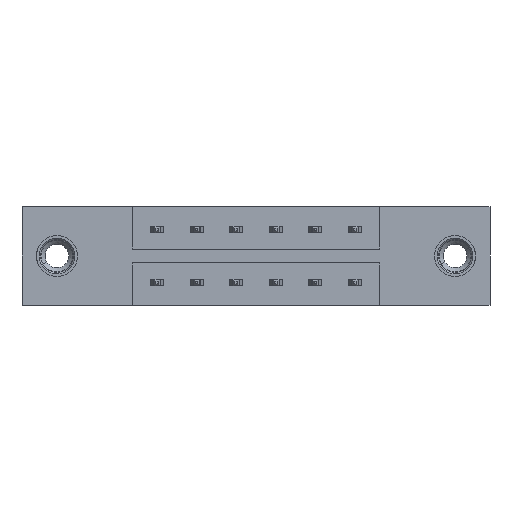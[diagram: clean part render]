
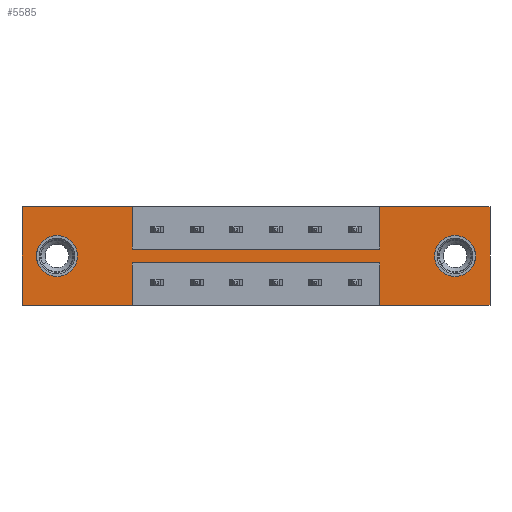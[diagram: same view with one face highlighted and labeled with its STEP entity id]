
A CAD part, front view. The second image highlights one B-rep face of the part: STEP entity #5585.
In plain terms, the highlighted planar face has unit normal (0, -1, 0).
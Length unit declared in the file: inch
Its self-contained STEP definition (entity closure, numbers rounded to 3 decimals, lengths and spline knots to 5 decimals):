
#4 = CARTESIAN_POINT ( 'NONE',  ( 1.775, 0., -0.375 ) ) ;
#118 = VERTEX_POINT ( 'NONE', #8989 ) ;
#135 = VECTOR ( 'NONE', #5515, 39.37008 ) ;
#169 = CIRCLE ( 'NONE', #7778, 0.078 ) ;
#213 = CARTESIAN_POINT ( 'NONE',  ( 0., 0., -0.375 ) ) ;
#219 = DIRECTION ( 'NONE',  ( 1., 0., 0. ) ) ;
#238 = VECTOR ( 'NONE', #4955, 39.37008 ) ;
#366 = DIRECTION ( 'NONE',  ( 0., 0., -1. ) ) ;
#485 = VECTOR ( 'NONE', #2483, 39.37008 ) ;
#530 = EDGE_CURVE ( 'NONE', #4576, #9027, #7301, .T. ) ;
#542 = ORIENTED_EDGE ( 'NONE', *, *, #5219, .F. ) ;
#544 = CARTESIAN_POINT ( 'NONE',  ( 1.6425, 0., -0.1875 ) ) ;
#625 = CARTESIAN_POINT ( 'NONE',  ( 0., 0., -0.375 ) ) ;
#694 = EDGE_CURVE ( 'NONE', #2834, #7868, #1300, .T. ) ;
#775 = CIRCLE ( 'NONE', #926, 0.078 ) ;
#806 = VERTEX_POINT ( 'NONE', #3602 ) ;
#830 = VECTOR ( 'NONE', #8016, 39.37008 ) ;
#875 = VECTOR ( 'NONE', #9648, 39.37008 ) ;
#926 = AXIS2_PLACEMENT_3D ( 'NONE', #544, #2720, #4322 ) ;
#1106 = AXIS2_PLACEMENT_3D ( 'NONE', #6571, #8780, #6470 ) ;
#1131 = ORIENTED_EDGE ( 'NONE', *, *, #530, .F. ) ;
#1161 = EDGE_LOOP ( 'NONE', ( #6562, #8916, #1131, #5868, #542, #4214, #4655, #4338, #6987, #3569, #9033, #2171 ) ) ;
#1178 = LINE ( 'NONE', #2723, #830 ) ;
#1208 = EDGE_CURVE ( 'NONE', #806, #8581, #5520, .T. ) ;
#1234 = EDGE_CURVE ( 'NONE', #5069, #4576, #1178, .T. ) ;
#1300 = LINE ( 'NONE', #625, #1649 ) ;
#1394 = VECTOR ( 'NONE', #366, 39.37008 ) ;
#1538 = VERTEX_POINT ( 'NONE', #7595 ) ;
#1649 = VECTOR ( 'NONE', #7380, 39.37008 ) ;
#1722 = CARTESIAN_POINT ( 'NONE',  ( 0., 0., 0. ) ) ;
#1952 = DIRECTION ( 'NONE',  ( 0., 1., 0. ) ) ;
#2171 = ORIENTED_EDGE ( 'NONE', *, *, #3201, .F. ) ;
#2472 = LINE ( 'NONE', #6971, #485 ) ;
#2483 = DIRECTION ( 'NONE',  ( 0., 0., 1. ) ) ;
#2505 = VERTEX_POINT ( 'NONE', #2828 ) ;
#2542 = VERTEX_POINT ( 'NONE', #7254 ) ;
#2720 = DIRECTION ( 'NONE',  ( 0., 1., 0. ) ) ;
#2723 = CARTESIAN_POINT ( 'NONE',  ( 0., 0., 0. ) ) ;
#2746 = LINE ( 'NONE', #4334, #5218 ) ;
#2828 = CARTESIAN_POINT ( 'NONE',  ( 1.6425, 0., -0.2655 ) ) ;
#2834 = VERTEX_POINT ( 'NONE', #4659 ) ;
#2861 = CARTESIAN_POINT ( 'NONE',  ( 1.775, 0., 0. ) ) ;
#2870 = LINE ( 'NONE', #9576, #875 ) ;
#2894 = AXIS2_PLACEMENT_3D ( 'NONE', #7270, #1952, #3412 ) ;
#2920 = AXIS2_PLACEMENT_3D ( 'NONE', #213, #7633, #7694 ) ;
#2939 = EDGE_CURVE ( 'NONE', #6679, #9699, #7095, .T. ) ;
#3072 = CARTESIAN_POINT ( 'NONE',  ( 0.4175, 0., 0. ) ) ;
#3193 = EDGE_CURVE ( 'NONE', #118, #2542, #2870, .T. ) ;
#3201 = EDGE_CURVE ( 'NONE', #2542, #4080, #5339, .T. ) ;
#3412 = DIRECTION ( 'NONE',  ( 0., 0., 1. ) ) ;
#3569 = ORIENTED_EDGE ( 'NONE', *, *, #694, .F. ) ;
#3581 = CARTESIAN_POINT ( 'NONE',  ( 0.4175, 0., -0.214 ) ) ;
#3602 = CARTESIAN_POINT ( 'NONE',  ( 0.1325, 0., -0.1095 ) ) ;
#3751 = EDGE_LOOP ( 'NONE', ( #9052, #9121 ) ) ;
#3846 = DIRECTION ( 'NONE',  ( 1., 0., 0. ) ) ;
#3864 = EDGE_CURVE ( 'NONE', #9699, #6518, #6841, .T. ) ;
#3989 = VERTEX_POINT ( 'NONE', #5786 ) ;
#4080 = VERTEX_POINT ( 'NONE', #4458 ) ;
#4113 = CARTESIAN_POINT ( 'NONE',  ( 1.775, 0., 0. ) ) ;
#4168 = DIRECTION ( 'NONE',  ( 0., 1., 0. ) ) ;
#4214 = ORIENTED_EDGE ( 'NONE', *, *, #7683, .F. ) ;
#4322 = DIRECTION ( 'NONE',  ( 0., 0., -1. ) ) ;
#4324 = VECTOR ( 'NONE', #3846, 39.37008 ) ;
#4334 = CARTESIAN_POINT ( 'NONE',  ( 0., 0., -0.375 ) ) ;
#4338 = ORIENTED_EDGE ( 'NONE', *, *, #2939, .F. ) ;
#4458 = CARTESIAN_POINT ( 'NONE',  ( 0.4175, 0., -0.214 ) ) ;
#4576 = VERTEX_POINT ( 'NONE', #2861 ) ;
#4655 = ORIENTED_EDGE ( 'NONE', *, *, #3864, .F. ) ;
#4659 = CARTESIAN_POINT ( 'NONE',  ( 0.4175, 0., -0.375 ) ) ;
#4712 = CARTESIAN_POINT ( 'NONE',  ( 0.1325, 0., -0.2655 ) ) ;
#4729 = CARTESIAN_POINT ( 'NONE',  ( 1.3575, 0., 0. ) ) ;
#4783 = EDGE_LOOP ( 'NONE', ( #7637, #8274 ) ) ;
#4851 = VECTOR ( 'NONE', #5842, 39.37008 ) ;
#4955 = DIRECTION ( 'NONE',  ( 0., 0., 1. ) ) ;
#5042 = LINE ( 'NONE', #9327, #1394 ) ;
#5069 = VERTEX_POINT ( 'NONE', #4729 ) ;
#5081 = EDGE_CURVE ( 'NONE', #7868, #6679, #2472, .T. ) ;
#5143 = CARTESIAN_POINT ( 'NONE',  ( 0.4175, 0., -0.161 ) ) ;
#5189 = LINE ( 'NONE', #7246, #238 ) ;
#5218 = VECTOR ( 'NONE', #8197, 39.37008 ) ;
#5219 = EDGE_CURVE ( 'NONE', #1538, #5069, #5189, .T. ) ;
#5339 = LINE ( 'NONE', #3581, #7563 ) ;
#5515 = DIRECTION ( 'NONE',  ( 0., 0., -1. ) ) ;
#5520 = CIRCLE ( 'NONE', #2894, 0.078 ) ;
#5585 = ADVANCED_FACE ( 'NONE', ( #9280, #7155, #7861 ), #6870, .T. ) ;
#5786 = CARTESIAN_POINT ( 'NONE',  ( 1.6425, 0., -0.1095 ) ) ;
#5842 = DIRECTION ( 'NONE',  ( 0., 0., -1. ) ) ;
#5868 = ORIENTED_EDGE ( 'NONE', *, *, #1234, .F. ) ;
#6352 = EDGE_CURVE ( 'NONE', #4080, #2834, #5042, .T. ) ;
#6370 = CARTESIAN_POINT ( 'NONE',  ( 0.1325, 0., -0.1875 ) ) ;
#6443 = DIRECTION ( 'NONE',  ( 0., 0., 1. ) ) ;
#6470 = DIRECTION ( 'NONE',  ( 0., 0., -1. ) ) ;
#6506 = DIRECTION ( 'NONE',  ( -1., 0., 0. ) ) ;
#6518 = VERTEX_POINT ( 'NONE', #8905 ) ;
#6562 = ORIENTED_EDGE ( 'NONE', *, *, #3193, .F. ) ;
#6571 = CARTESIAN_POINT ( 'NONE',  ( 1.6425, 0., -0.1875 ) ) ;
#6679 = VERTEX_POINT ( 'NONE', #7517 ) ;
#6841 = LINE ( 'NONE', #5143, #4851 ) ;
#6870 = PLANE ( 'NONE',  #2920 ) ;
#6971 = CARTESIAN_POINT ( 'NONE',  ( 0., 0., 0. ) ) ;
#6987 = ORIENTED_EDGE ( 'NONE', *, *, #5081, .F. ) ;
#7095 = LINE ( 'NONE', #1722, #9696 ) ;
#7155 = FACE_BOUND ( 'NONE', #3751, .T. ) ;
#7246 = CARTESIAN_POINT ( 'NONE',  ( 1.3575, 0., -0.161 ) ) ;
#7254 = CARTESIAN_POINT ( 'NONE',  ( 1.3575, 0., -0.214 ) ) ;
#7270 = CARTESIAN_POINT ( 'NONE',  ( 0.1325, 0., -0.1875 ) ) ;
#7301 = LINE ( 'NONE', #4113, #135 ) ;
#7374 = CARTESIAN_POINT ( 'NONE',  ( 0.4175, 0., -0.161 ) ) ;
#7380 = DIRECTION ( 'NONE',  ( -1., 0., 0. ) ) ;
#7517 = CARTESIAN_POINT ( 'NONE',  ( 0., 0., 0. ) ) ;
#7563 = VECTOR ( 'NONE', #6506, 39.37008 ) ;
#7595 = CARTESIAN_POINT ( 'NONE',  ( 1.3575, 0., -0.161 ) ) ;
#7633 = DIRECTION ( 'NONE',  ( 0., -1., 0. ) ) ;
#7637 = ORIENTED_EDGE ( 'NONE', *, *, #8062, .T. ) ;
#7683 = EDGE_CURVE ( 'NONE', #6518, #1538, #8891, .T. ) ;
#7694 = DIRECTION ( 'NONE',  ( 0., 0., -1. ) ) ;
#7778 = AXIS2_PLACEMENT_3D ( 'NONE', #6370, #4168, #6443 ) ;
#7861 = FACE_OUTER_BOUND ( 'NONE', #1161, .T. ) ;
#7868 = VERTEX_POINT ( 'NONE', #9213 ) ;
#8016 = DIRECTION ( 'NONE',  ( 1., 0., 0. ) ) ;
#8062 = EDGE_CURVE ( 'NONE', #3989, #2505, #775, .T. ) ;
#8093 = EDGE_CURVE ( 'NONE', #2505, #3989, #8164, .T. ) ;
#8164 = CIRCLE ( 'NONE', #1106, 0.078 ) ;
#8197 = DIRECTION ( 'NONE',  ( -1., 0., 0. ) ) ;
#8274 = ORIENTED_EDGE ( 'NONE', *, *, #8093, .T. ) ;
#8581 = VERTEX_POINT ( 'NONE', #4712 ) ;
#8780 = DIRECTION ( 'NONE',  ( 0., 1., 0. ) ) ;
#8891 = LINE ( 'NONE', #7374, #4324 ) ;
#8905 = CARTESIAN_POINT ( 'NONE',  ( 0.4175, 0., -0.161 ) ) ;
#8916 = ORIENTED_EDGE ( 'NONE', *, *, #9556, .F. ) ;
#8989 = CARTESIAN_POINT ( 'NONE',  ( 1.3575, 0., -0.375 ) ) ;
#9027 = VERTEX_POINT ( 'NONE', #4 ) ;
#9033 = ORIENTED_EDGE ( 'NONE', *, *, #6352, .F. ) ;
#9052 = ORIENTED_EDGE ( 'NONE', *, *, #1208, .T. ) ;
#9121 = ORIENTED_EDGE ( 'NONE', *, *, #9354, .T. ) ;
#9213 = CARTESIAN_POINT ( 'NONE',  ( 0., 0., -0.375 ) ) ;
#9280 = FACE_BOUND ( 'NONE', #4783, .T. ) ;
#9327 = CARTESIAN_POINT ( 'NONE',  ( 0.4175, 0., -0.214 ) ) ;
#9354 = EDGE_CURVE ( 'NONE', #8581, #806, #169, .T. ) ;
#9556 = EDGE_CURVE ( 'NONE', #9027, #118, #2746, .T. ) ;
#9576 = CARTESIAN_POINT ( 'NONE',  ( 1.3575, 0., -0.214 ) ) ;
#9648 = DIRECTION ( 'NONE',  ( 0., 0., 1. ) ) ;
#9696 = VECTOR ( 'NONE', #219, 39.37008 ) ;
#9699 = VERTEX_POINT ( 'NONE', #3072 ) ;
